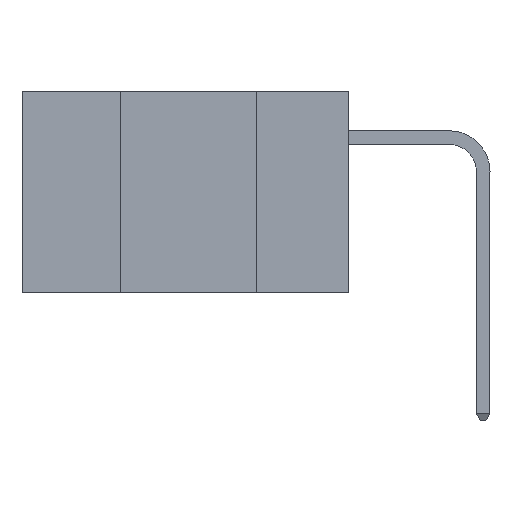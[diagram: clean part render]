
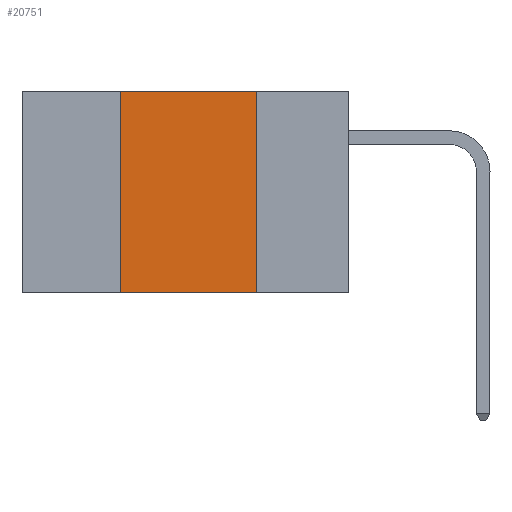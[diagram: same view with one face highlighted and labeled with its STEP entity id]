
A CAD part, left-side view. The second image highlights one B-rep face of the part: STEP entity #20751.
In plain terms, the highlighted planar face has unit normal (-1, 0, 0).
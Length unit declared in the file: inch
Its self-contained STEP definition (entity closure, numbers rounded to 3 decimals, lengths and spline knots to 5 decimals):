
#46 = CARTESIAN_POINT ( 'NONE',  ( 0., 0.42, 0. ) ) ;
#78 = VECTOR ( 'NONE', #13883, 39.37008 ) ;
#288 = VECTOR ( 'NONE', #339, 39.37008 ) ;
#339 = DIRECTION ( 'NONE',  ( 0., -1., 0. ) ) ;
#534 = EDGE_CURVE ( 'NONE', #19399, #10423, #20055, .T. ) ;
#4316 = EDGE_LOOP ( 'NONE', ( #13761, #19218, #10215, #16216 ) ) ;
#5013 = LINE ( 'NONE', #17472, #78 ) ;
#6166 = AXIS2_PLACEMENT_3D ( 'NONE', #18594, #20406, #9486 ) ;
#6943 = DIRECTION ( 'NONE',  ( 0., 0., -1. ) ) ;
#7696 = LINE ( 'NONE', #18781, #12041 ) ;
#8129 = EDGE_CURVE ( 'NONE', #19038, #12262, #5013, .T. ) ;
#9486 = DIRECTION ( 'NONE',  ( 0., 0., -1. ) ) ;
#10215 = ORIENTED_EDGE ( 'NONE', *, *, #8129, .F. ) ;
#10423 = VERTEX_POINT ( 'NONE', #18566 ) ;
#11284 = PLANE ( 'NONE',  #6166 ) ;
#11405 = FACE_OUTER_BOUND ( 'NONE', #4316, .T. ) ;
#12041 = VECTOR ( 'NONE', #20601, 39.37008 ) ;
#12262 = VERTEX_POINT ( 'NONE', #46 ) ;
#13761 = ORIENTED_EDGE ( 'NONE', *, *, #534, .F. ) ;
#13883 = DIRECTION ( 'NONE',  ( 0., 0., 1. ) ) ;
#15017 = LINE ( 'NONE', #22329, #288 ) ;
#16216 = ORIENTED_EDGE ( 'NONE', *, *, #22083, .T. ) ;
#16257 = EDGE_CURVE ( 'NONE', #12262, #19399, #7696, .T. ) ;
#17472 = CARTESIAN_POINT ( 'NONE',  ( 0., 0.42, 0. ) ) ;
#18566 = CARTESIAN_POINT ( 'NONE',  ( 0., 0.17, -0.37 ) ) ;
#18594 = CARTESIAN_POINT ( 'NONE',  ( 0., 0.6, 0. ) ) ;
#18781 = CARTESIAN_POINT ( 'NONE',  ( 0., 0.6, 0. ) ) ;
#18896 = CARTESIAN_POINT ( 'NONE',  ( 0., 0.42, -0.37 ) ) ;
#19038 = VERTEX_POINT ( 'NONE', #18896 ) ;
#19218 = ORIENTED_EDGE ( 'NONE', *, *, #16257, .F. ) ;
#19399 = VERTEX_POINT ( 'NONE', #21633 ) ;
#19494 = VECTOR ( 'NONE', #6943, 39.37008 ) ;
#19680 = CARTESIAN_POINT ( 'NONE',  ( 0., 0.17, 0. ) ) ;
#20055 = LINE ( 'NONE', #19680, #19494 ) ;
#20406 = DIRECTION ( 'NONE',  ( 1., 0., 0. ) ) ;
#20601 = DIRECTION ( 'NONE',  ( 0., -1., 0. ) ) ;
#20751 = ADVANCED_FACE ( 'NONE', ( #11405 ), #11284, .F. ) ;
#21633 = CARTESIAN_POINT ( 'NONE',  ( 0., 0.17, 0. ) ) ;
#22083 = EDGE_CURVE ( 'NONE', #19038, #10423, #15017, .T. ) ;
#22329 = CARTESIAN_POINT ( 'NONE',  ( 0., 0.6, -0.37 ) ) ;
